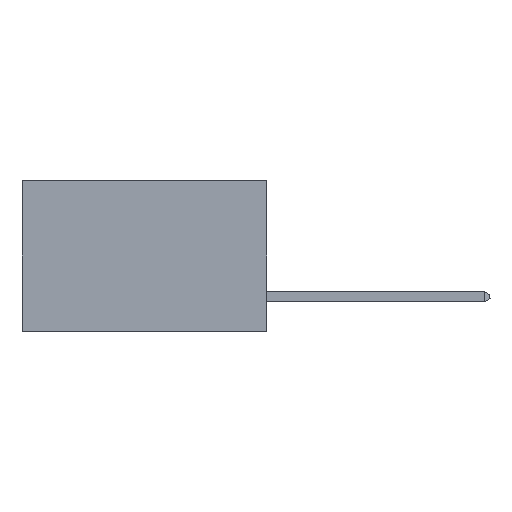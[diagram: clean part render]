
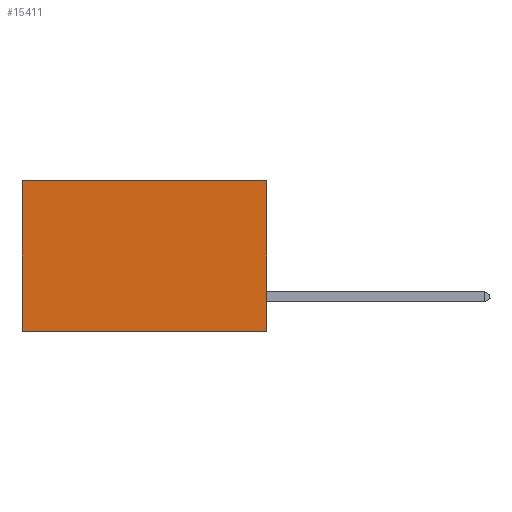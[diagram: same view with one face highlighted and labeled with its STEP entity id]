
A CAD part, left-side view. The second image highlights one B-rep face of the part: STEP entity #15411.
In plain terms, the highlighted planar face has unit normal (-1, 0, 0).
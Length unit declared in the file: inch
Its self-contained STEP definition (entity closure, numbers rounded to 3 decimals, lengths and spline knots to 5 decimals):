
#424 = CARTESIAN_POINT ( 'NONE',  ( 0.2875, 0., -0.37 ) ) ;
#1302 = DIRECTION ( 'NONE',  ( 0., 0., -1. ) ) ;
#3282 = AXIS2_PLACEMENT_3D ( 'NONE', #11119, #5632, #1302 ) ;
#3361 = ORIENTED_EDGE ( 'NONE', *, *, #17655, .T. ) ;
#3372 = LINE ( 'NONE', #424, #24162 ) ;
#4489 = LINE ( 'NONE', #24319, #22647 ) ;
#5181 = CARTESIAN_POINT ( 'NONE',  ( 0.2875, 0., 0. ) ) ;
#5632 = DIRECTION ( 'NONE',  ( 1., 0., 0. ) ) ;
#7595 = VERTEX_POINT ( 'NONE', #27172 ) ;
#7751 = CARTESIAN_POINT ( 'NONE',  ( 0.2875, 0., -0.37 ) ) ;
#8177 = EDGE_CURVE ( 'NONE', #17997, #15958, #3372, .T. ) ;
#8439 = ORIENTED_EDGE ( 'NONE', *, *, #8177, .F. ) ;
#10327 = EDGE_CURVE ( 'NONE', #28640, #7595, #15365, .T. ) ;
#11119 = CARTESIAN_POINT ( 'NONE',  ( 0.2875, 0., 0. ) ) ;
#12283 = DIRECTION ( 'NONE',  ( 0., 1., 0. ) ) ;
#12464 = DIRECTION ( 'NONE',  ( 0., 0., -1. ) ) ;
#13661 = CARTESIAN_POINT ( 'NONE',  ( 0.2875, 0., 0. ) ) ;
#15365 = LINE ( 'NONE', #5181, #20242 ) ;
#15411 = ADVANCED_FACE ( 'NONE', ( #24987 ), #19751, .F. ) ;
#15958 = VERTEX_POINT ( 'NONE', #31228 ) ;
#16691 = EDGE_LOOP ( 'NONE', ( #3361, #8439, #25258, #28569 ) ) ;
#17264 = DIRECTION ( 'NONE',  ( 0., 0., -1. ) ) ;
#17655 = EDGE_CURVE ( 'NONE', #7595, #15958, #29804, .T. ) ;
#17997 = VERTEX_POINT ( 'NONE', #7751 ) ;
#19751 = PLANE ( 'NONE',  #3282 ) ;
#19941 = EDGE_CURVE ( 'NONE', #28640, #17997, #4489, .T. ) ;
#20242 = VECTOR ( 'NONE', #27087, 39.37008 ) ;
#21043 = VECTOR ( 'NONE', #12464, 39.37008 ) ;
#21845 = CARTESIAN_POINT ( 'NONE',  ( 0.2875, 0.6, 0. ) ) ;
#22647 = VECTOR ( 'NONE', #17264, 39.37008 ) ;
#24162 = VECTOR ( 'NONE', #12283, 39.37008 ) ;
#24319 = CARTESIAN_POINT ( 'NONE',  ( 0.2875, 0., 0. ) ) ;
#24987 = FACE_OUTER_BOUND ( 'NONE', #16691, .T. ) ;
#25258 = ORIENTED_EDGE ( 'NONE', *, *, #19941, .F. ) ;
#27087 = DIRECTION ( 'NONE',  ( 0., 1., 0. ) ) ;
#27172 = CARTESIAN_POINT ( 'NONE',  ( 0.2875, 0.6, 0. ) ) ;
#28569 = ORIENTED_EDGE ( 'NONE', *, *, #10327, .T. ) ;
#28640 = VERTEX_POINT ( 'NONE', #13661 ) ;
#29804 = LINE ( 'NONE', #21845, #21043 ) ;
#31228 = CARTESIAN_POINT ( 'NONE',  ( 0.2875, 0.6, -0.37 ) ) ;
